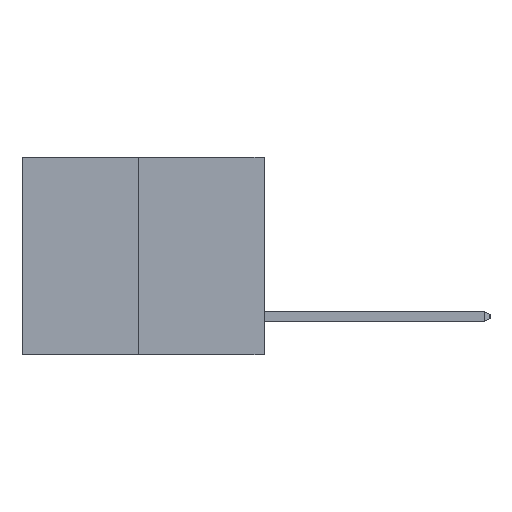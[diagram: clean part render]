
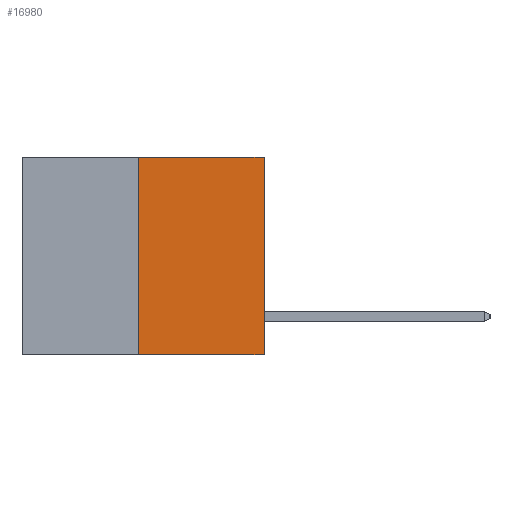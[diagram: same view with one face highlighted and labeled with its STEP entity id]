
A CAD part, left-side view. The second image highlights one B-rep face of the part: STEP entity #16980.
In plain terms, the highlighted planar face has unit normal (-1, 0, 0).
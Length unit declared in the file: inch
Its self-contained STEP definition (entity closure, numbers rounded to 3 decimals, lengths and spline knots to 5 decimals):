
#98 = VECTOR ( 'NONE', #6241, 39.37008 ) ;
#273 = LINE ( 'NONE', #15898, #3368 ) ;
#566 = CARTESIAN_POINT ( 'NONE',  ( 0., 0., 0. ) ) ;
#1044 = FACE_OUTER_BOUND ( 'NONE', #12571, .T. ) ;
#1396 = CARTESIAN_POINT ( 'NONE',  ( 0., 0.312, 0. ) ) ;
#1705 = ORIENTED_EDGE ( 'NONE', *, *, #4555, .T. ) ;
#2570 = LINE ( 'NONE', #14178, #98 ) ;
#2593 = DIRECTION ( 'NONE',  ( 0., -1., 0. ) ) ;
#2668 = VERTEX_POINT ( 'NONE', #1396 ) ;
#3368 = VECTOR ( 'NONE', #5264, 39.37008 ) ;
#3507 = AXIS2_PLACEMENT_3D ( 'NONE', #3612, #4997, #15625 ) ;
#3612 = CARTESIAN_POINT ( 'NONE',  ( 0., 0.6, 0. ) ) ;
#4074 = CARTESIAN_POINT ( 'NONE',  ( 0., 0., -0.49 ) ) ;
#4555 = EDGE_CURVE ( 'NONE', #6826, #15601, #2570, .T. ) ;
#4997 = DIRECTION ( 'NONE',  ( 1., 0., 0. ) ) ;
#5264 = DIRECTION ( 'NONE',  ( 0., -1., 0. ) ) ;
#5363 = DIRECTION ( 'NONE',  ( 0., 0., 1. ) ) ;
#6145 = PLANE ( 'NONE',  #3507 ) ;
#6241 = DIRECTION ( 'NONE',  ( 0., 0., 1. ) ) ;
#6826 = VERTEX_POINT ( 'NONE', #4074 ) ;
#7402 = CARTESIAN_POINT ( 'NONE',  ( 0., 0.312, -0.49 ) ) ;
#9236 = CARTESIAN_POINT ( 'NONE',  ( 0., 0.312, -0.49 ) ) ;
#9314 = EDGE_CURVE ( 'NONE', #10760, #2668, #15951, .T. ) ;
#10686 = ORIENTED_EDGE ( 'NONE', *, *, #15120, .T. ) ;
#10760 = VERTEX_POINT ( 'NONE', #7402 ) ;
#10825 = ORIENTED_EDGE ( 'NONE', *, *, #9314, .F. ) ;
#10879 = ORIENTED_EDGE ( 'NONE', *, *, #15108, .F. ) ;
#11313 = LINE ( 'NONE', #14756, #14467 ) ;
#12433 = VECTOR ( 'NONE', #5363, 39.37008 ) ;
#12571 = EDGE_LOOP ( 'NONE', ( #10825, #10686, #1705, #10879 ) ) ;
#14178 = CARTESIAN_POINT ( 'NONE',  ( 0., 0., 0. ) ) ;
#14467 = VECTOR ( 'NONE', #2593, 39.37008 ) ;
#14756 = CARTESIAN_POINT ( 'NONE',  ( 0., 0.6, 0. ) ) ;
#15108 = EDGE_CURVE ( 'NONE', #2668, #15601, #11313, .T. ) ;
#15120 = EDGE_CURVE ( 'NONE', #10760, #6826, #273, .T. ) ;
#15601 = VERTEX_POINT ( 'NONE', #566 ) ;
#15625 = DIRECTION ( 'NONE',  ( 0., 0., -1. ) ) ;
#15898 = CARTESIAN_POINT ( 'NONE',  ( 0., 0.6, -0.49 ) ) ;
#15951 = LINE ( 'NONE', #9236, #12433 ) ;
#16980 = ADVANCED_FACE ( 'NONE', ( #1044 ), #6145, .F. ) ;
